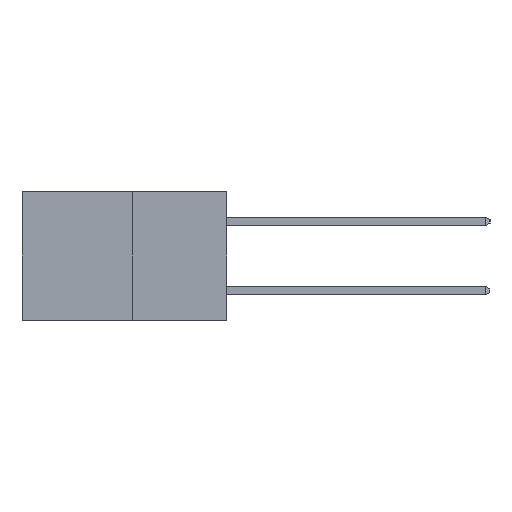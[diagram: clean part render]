
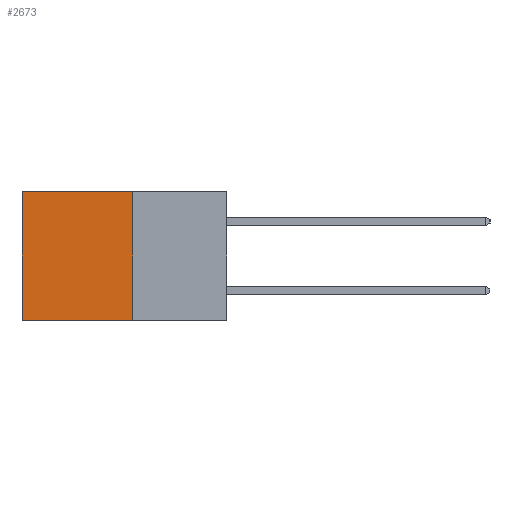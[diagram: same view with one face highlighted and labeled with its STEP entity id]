
A CAD part, left-side view. The second image highlights one B-rep face of the part: STEP entity #2673.
In plain terms, the highlighted planar face has unit normal (-1, 0, 0).
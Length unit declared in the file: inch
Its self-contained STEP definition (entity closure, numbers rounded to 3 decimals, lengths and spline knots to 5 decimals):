
#337 = ORIENTED_EDGE ( 'NONE', *, *, #3791, .F. ) ;
#1290 = CARTESIAN_POINT ( 'NONE',  ( 0.277, 0.27, 0. ) ) ;
#1593 = CARTESIAN_POINT ( 'NONE',  ( 0.277, 0.59, 0. ) ) ;
#2673 = ADVANCED_FACE ( 'NONE', ( #6407 ), #10212, .F. ) ;
#2848 = DIRECTION ( 'NONE',  ( 0., 0., -1. ) ) ;
#3002 = AXIS2_PLACEMENT_3D ( 'NONE', #10980, #9770, #9768 ) ;
#3522 = VECTOR ( 'NONE', #2848, 39.37008 ) ;
#3598 = CARTESIAN_POINT ( 'NONE',  ( 0.277, 0.27, 0. ) ) ;
#3777 = DIRECTION ( 'NONE',  ( 0., 1., 0. ) ) ;
#3791 = EDGE_CURVE ( 'NONE', #8111, #4937, #5547, .T. ) ;
#3832 = LINE ( 'NONE', #10926, #3522 ) ;
#3854 = CARTESIAN_POINT ( 'NONE',  ( 0.277, 0.27, -0.37 ) ) ;
#4028 = EDGE_CURVE ( 'NONE', #8725, #5951, #11483, .T. ) ;
#4176 = CARTESIAN_POINT ( 'NONE',  ( 0.277, 0.59, -0.37 ) ) ;
#4634 = LINE ( 'NONE', #8237, #8839 ) ;
#4816 = VECTOR ( 'NONE', #3777, 39.37008 ) ;
#4937 = VERTEX_POINT ( 'NONE', #4176 ) ;
#5547 = LINE ( 'NONE', #3854, #7915 ) ;
#5951 = VERTEX_POINT ( 'NONE', #1593 ) ;
#6407 = FACE_OUTER_BOUND ( 'NONE', #10034, .T. ) ;
#6633 = ORIENTED_EDGE ( 'NONE', *, *, #7966, .F. ) ;
#7915 = VECTOR ( 'NONE', #8705, 39.37008 ) ;
#7966 = EDGE_CURVE ( 'NONE', #8725, #8111, #4634, .T. ) ;
#8111 = VERTEX_POINT ( 'NONE', #10907 ) ;
#8237 = CARTESIAN_POINT ( 'NONE',  ( 0.277, 0.27, -0.37 ) ) ;
#8705 = DIRECTION ( 'NONE',  ( 0., 1., 0. ) ) ;
#8725 = VERTEX_POINT ( 'NONE', #3598 ) ;
#8839 = VECTOR ( 'NONE', #9129, 39.37008 ) ;
#9017 = EDGE_CURVE ( 'NONE', #5951, #4937, #3832, .T. ) ;
#9129 = DIRECTION ( 'NONE',  ( 0., 0., -1. ) ) ;
#9768 = DIRECTION ( 'NONE',  ( 0., 0., -1. ) ) ;
#9770 = DIRECTION ( 'NONE',  ( 1., 0., 0. ) ) ;
#10034 = EDGE_LOOP ( 'NONE', ( #11339, #337, #6633, #11742 ) ) ;
#10212 = PLANE ( 'NONE',  #3002 ) ;
#10907 = CARTESIAN_POINT ( 'NONE',  ( 0.277, 0.27, -0.37 ) ) ;
#10926 = CARTESIAN_POINT ( 'NONE',  ( 0.277, 0.59, -0.37 ) ) ;
#10980 = CARTESIAN_POINT ( 'NONE',  ( 0.277, 0.27, -0.37 ) ) ;
#11339 = ORIENTED_EDGE ( 'NONE', *, *, #9017, .T. ) ;
#11483 = LINE ( 'NONE', #1290, #4816 ) ;
#11742 = ORIENTED_EDGE ( 'NONE', *, *, #4028, .T. ) ;
